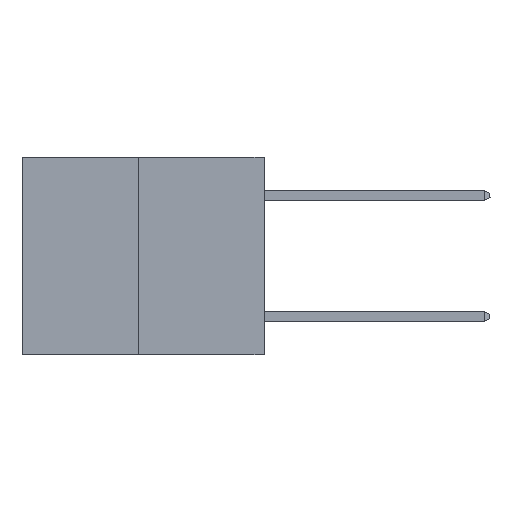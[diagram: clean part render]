
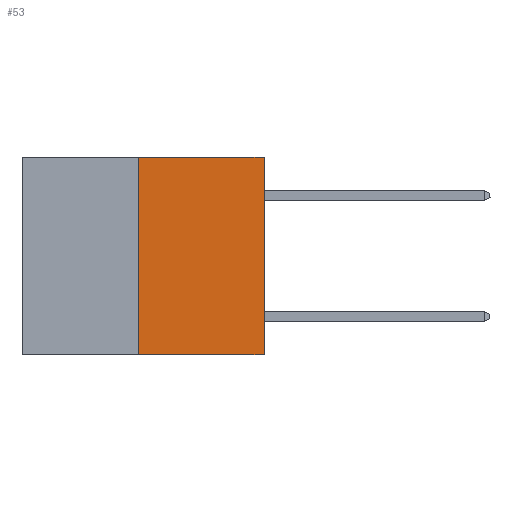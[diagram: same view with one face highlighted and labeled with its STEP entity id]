
A CAD part, left-side view. The second image highlights one B-rep face of the part: STEP entity #53.
In plain terms, the highlighted planar face has unit normal (-1, 0, 0).
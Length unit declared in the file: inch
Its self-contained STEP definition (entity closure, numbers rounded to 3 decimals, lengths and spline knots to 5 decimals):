
#53 = ADVANCED_FACE ( 'NONE', ( #5592 ), #5986, .F. ) ;
#1251 = VECTOR ( 'NONE', #11566, 39.37008 ) ;
#1678 = EDGE_LOOP ( 'NONE', ( #16334, #4533, #11868, #6490 ) ) ;
#1941 = CARTESIAN_POINT ( 'NONE',  ( 0., 0., -0.49 ) ) ;
#1946 = EDGE_CURVE ( 'NONE', #8934, #15911, #5973, .T. ) ;
#2036 = DIRECTION ( 'NONE',  ( 0., 0., 1. ) ) ;
#4031 = CARTESIAN_POINT ( 'NONE',  ( 0., 0.312, -0.49 ) ) ;
#4171 = VERTEX_POINT ( 'NONE', #1941 ) ;
#4533 = ORIENTED_EDGE ( 'NONE', *, *, #11481, .T. ) ;
#5592 = FACE_OUTER_BOUND ( 'NONE', #1678, .T. ) ;
#5609 = CARTESIAN_POINT ( 'NONE',  ( 0., 0.6, 0. ) ) ;
#5973 = LINE ( 'NONE', #4031, #9696 ) ;
#5986 = PLANE ( 'NONE',  #12742 ) ;
#6109 = LINE ( 'NONE', #11597, #1251 ) ;
#6490 = ORIENTED_EDGE ( 'NONE', *, *, #17925, .F. ) ;
#7767 = DIRECTION ( 'NONE',  ( 1., 0., 0. ) ) ;
#8934 = VERTEX_POINT ( 'NONE', #21408 ) ;
#9696 = VECTOR ( 'NONE', #2036, 39.37008 ) ;
#11481 = EDGE_CURVE ( 'NONE', #8934, #4171, #12471, .T. ) ;
#11566 = DIRECTION ( 'NONE',  ( 0., 0., 1. ) ) ;
#11597 = CARTESIAN_POINT ( 'NONE',  ( 0., 0., 0. ) ) ;
#11868 = ORIENTED_EDGE ( 'NONE', *, *, #22287, .T. ) ;
#12471 = LINE ( 'NONE', #22878, #16156 ) ;
#12742 = AXIS2_PLACEMENT_3D ( 'NONE', #18737, #7767, #22403 ) ;
#13918 = CARTESIAN_POINT ( 'NONE',  ( 0., 0.312, 0. ) ) ;
#14848 = DIRECTION ( 'NONE',  ( 0., -1., 0. ) ) ;
#15621 = DIRECTION ( 'NONE',  ( 0., -1., 0. ) ) ;
#15911 = VERTEX_POINT ( 'NONE', #13918 ) ;
#16156 = VECTOR ( 'NONE', #15621, 39.37008 ) ;
#16334 = ORIENTED_EDGE ( 'NONE', *, *, #1946, .F. ) ;
#17925 = EDGE_CURVE ( 'NONE', #15911, #23025, #18342, .T. ) ;
#18342 = LINE ( 'NONE', #5609, #22624 ) ;
#18737 = CARTESIAN_POINT ( 'NONE',  ( 0., 0.6, 0. ) ) ;
#21408 = CARTESIAN_POINT ( 'NONE',  ( 0., 0.312, -0.49 ) ) ;
#22287 = EDGE_CURVE ( 'NONE', #4171, #23025, #6109, .T. ) ;
#22403 = DIRECTION ( 'NONE',  ( 0., 0., -1. ) ) ;
#22624 = VECTOR ( 'NONE', #14848, 39.37008 ) ;
#22878 = CARTESIAN_POINT ( 'NONE',  ( 0., 0.6, -0.49 ) ) ;
#23025 = VERTEX_POINT ( 'NONE', #23277 ) ;
#23277 = CARTESIAN_POINT ( 'NONE',  ( 0., 0., 0. ) ) ;
